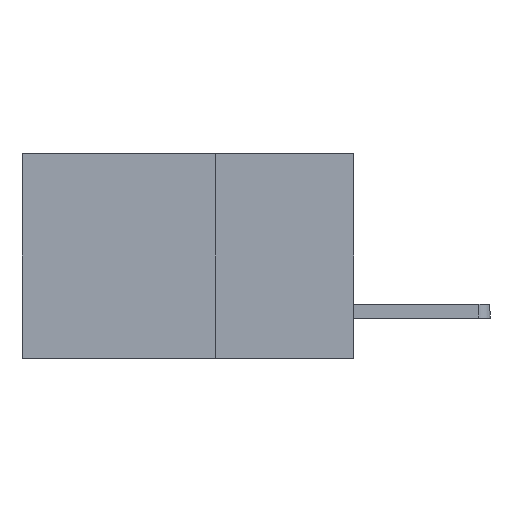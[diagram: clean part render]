
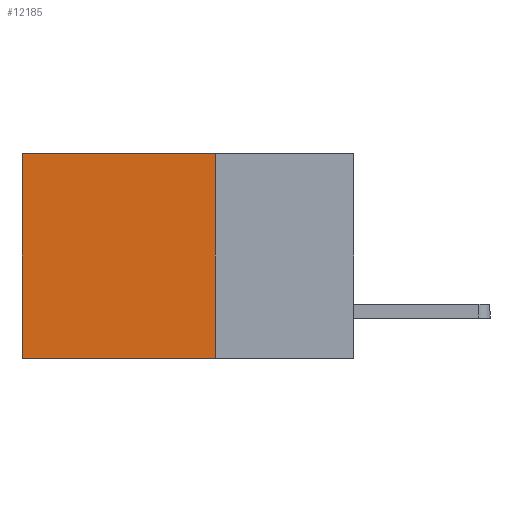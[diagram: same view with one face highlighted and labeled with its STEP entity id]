
A CAD part, left-side view. The second image highlights one B-rep face of the part: STEP entity #12185.
In plain terms, the highlighted planar face has unit normal (-1, 0, 0).
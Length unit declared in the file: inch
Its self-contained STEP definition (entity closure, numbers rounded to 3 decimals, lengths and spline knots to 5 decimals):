
#390 = LINE ( 'NONE', #3952, #6496 ) ;
#605 = FACE_OUTER_BOUND ( 'NONE', #4751, .T. ) ;
#644 = CARTESIAN_POINT ( 'NONE',  ( 0.2875, 0.25, 0. ) ) ;
#1054 = VECTOR ( 'NONE', #2415, 39.37008 ) ;
#1253 = LINE ( 'NONE', #4514, #12712 ) ;
#1760 = DIRECTION ( 'NONE',  ( 0., 0., -1. ) ) ;
#1796 = CARTESIAN_POINT ( 'NONE',  ( 0.2875, 0.25, 0. ) ) ;
#2415 = DIRECTION ( 'NONE',  ( 0., 1., 0. ) ) ;
#2869 = VECTOR ( 'NONE', #10350, 39.37008 ) ;
#2874 = ORIENTED_EDGE ( 'NONE', *, *, #3385, .F. ) ;
#3066 = CARTESIAN_POINT ( 'NONE',  ( 0.2875, 0.25, -0.37 ) ) ;
#3385 = EDGE_CURVE ( 'NONE', #12848, #10768, #390, .T. ) ;
#3952 = CARTESIAN_POINT ( 'NONE',  ( 0.2875, 0.25, 0. ) ) ;
#4514 = CARTESIAN_POINT ( 'NONE',  ( 0.2875, 0.6, 0. ) ) ;
#4751 = EDGE_LOOP ( 'NONE', ( #13296, #12854, #2874, #6000 ) ) ;
#5113 = VERTEX_POINT ( 'NONE', #12728 ) ;
#6000 = ORIENTED_EDGE ( 'NONE', *, *, #8452, .T. ) ;
#6490 = VERTEX_POINT ( 'NONE', #11670 ) ;
#6496 = VECTOR ( 'NONE', #7099, 39.37008 ) ;
#6723 = CARTESIAN_POINT ( 'NONE',  ( 0.2875, 0.25, 0. ) ) ;
#6943 = EDGE_CURVE ( 'NONE', #10768, #6490, #11236, .T. ) ;
#7085 = PLANE ( 'NONE',  #11694 ) ;
#7099 = DIRECTION ( 'NONE',  ( 0., 0., -1. ) ) ;
#7833 = EDGE_CURVE ( 'NONE', #5113, #6490, #1253, .T. ) ;
#8160 = DIRECTION ( 'NONE',  ( 1., 0., 0. ) ) ;
#8452 = EDGE_CURVE ( 'NONE', #12848, #5113, #12213, .T. ) ;
#9365 = CARTESIAN_POINT ( 'NONE',  ( 0.2875, 0.25, -0.37 ) ) ;
#10350 = DIRECTION ( 'NONE',  ( 0., 1., 0. ) ) ;
#10768 = VERTEX_POINT ( 'NONE', #3066 ) ;
#11236 = LINE ( 'NONE', #9365, #2869 ) ;
#11670 = CARTESIAN_POINT ( 'NONE',  ( 0.2875, 0.6, -0.37 ) ) ;
#11694 = AXIS2_PLACEMENT_3D ( 'NONE', #644, #8160, #1760 ) ;
#11771 = DIRECTION ( 'NONE',  ( 0., 0., -1. ) ) ;
#12185 = ADVANCED_FACE ( 'NONE', ( #605 ), #7085, .F. ) ;
#12213 = LINE ( 'NONE', #6723, #1054 ) ;
#12712 = VECTOR ( 'NONE', #11771, 39.37008 ) ;
#12728 = CARTESIAN_POINT ( 'NONE',  ( 0.2875, 0.6, 0. ) ) ;
#12848 = VERTEX_POINT ( 'NONE', #1796 ) ;
#12854 = ORIENTED_EDGE ( 'NONE', *, *, #6943, .F. ) ;
#13296 = ORIENTED_EDGE ( 'NONE', *, *, #7833, .T. ) ;
